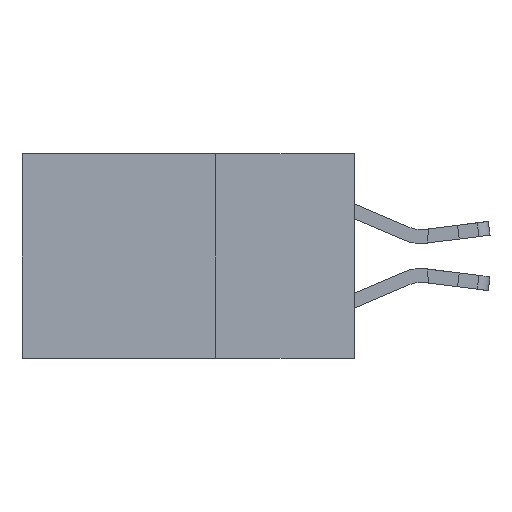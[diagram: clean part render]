
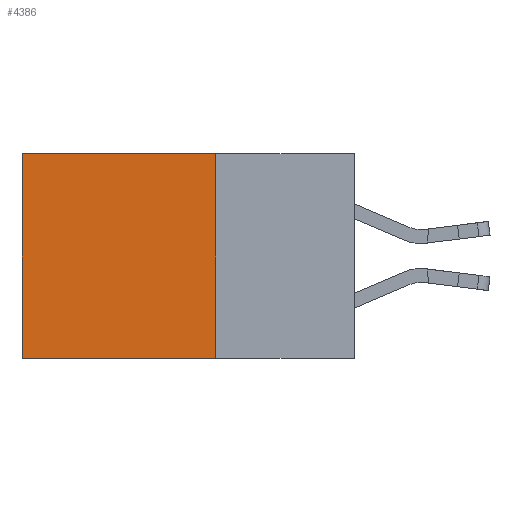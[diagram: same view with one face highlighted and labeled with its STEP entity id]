
A CAD part, left-side view. The second image highlights one B-rep face of the part: STEP entity #4386.
In plain terms, the highlighted planar face has unit normal (-1, 0, 0).
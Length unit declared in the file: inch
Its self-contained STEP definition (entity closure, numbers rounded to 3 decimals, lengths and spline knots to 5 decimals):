
#367 = DIRECTION ( 'NONE',  ( 0., 0., -1. ) ) ;
#418 = AXIS2_PLACEMENT_3D ( 'NONE', #9059, #8296, #367 ) ;
#1552 = DIRECTION ( 'NONE',  ( 0., 0., -1. ) ) ;
#1783 = LINE ( 'NONE', #6943, #2686 ) ;
#2231 = CARTESIAN_POINT ( 'NONE',  ( 0.2615, 0.25, -0.37 ) ) ;
#2245 = LINE ( 'NONE', #2784, #10789 ) ;
#2415 = CARTESIAN_POINT ( 'NONE',  ( 0.2615, 0.6, -0.37 ) ) ;
#2583 = VECTOR ( 'NONE', #1552, 39.37008 ) ;
#2585 = VERTEX_POINT ( 'NONE', #7213 ) ;
#2609 = EDGE_CURVE ( 'NONE', #7140, #4555, #1783, .T. ) ;
#2686 = VECTOR ( 'NONE', #7809, 39.37008 ) ;
#2784 = CARTESIAN_POINT ( 'NONE',  ( 0.2615, 0.25, -0.37 ) ) ;
#3113 = LINE ( 'NONE', #2231, #7549 ) ;
#3255 = CARTESIAN_POINT ( 'NONE',  ( 0.2615, 0.25, 0. ) ) ;
#3738 = ORIENTED_EDGE ( 'NONE', *, *, #10870, .F. ) ;
#4386 = ADVANCED_FACE ( 'NONE', ( #9820 ), #7427, .F. ) ;
#4390 = ORIENTED_EDGE ( 'NONE', *, *, #2609, .T. ) ;
#4555 = VERTEX_POINT ( 'NONE', #4958 ) ;
#4958 = CARTESIAN_POINT ( 'NONE',  ( 0.2615, 0.6, 0. ) ) ;
#5749 = VERTEX_POINT ( 'NONE', #9417 ) ;
#6943 = CARTESIAN_POINT ( 'NONE',  ( 0.2615, 0.25, 0. ) ) ;
#7140 = VERTEX_POINT ( 'NONE', #3255 ) ;
#7213 = CARTESIAN_POINT ( 'NONE',  ( 0.2615, 0.6, -0.37 ) ) ;
#7427 = PLANE ( 'NONE',  #418 ) ;
#7490 = ORIENTED_EDGE ( 'NONE', *, *, #10914, .T. ) ;
#7549 = VECTOR ( 'NONE', #9359, 39.37008 ) ;
#7809 = DIRECTION ( 'NONE',  ( 0., 1., 0. ) ) ;
#8188 = EDGE_CURVE ( 'NONE', #7140, #5749, #2245, .T. ) ;
#8296 = DIRECTION ( 'NONE',  ( 1., 0., 0. ) ) ;
#8417 = ORIENTED_EDGE ( 'NONE', *, *, #8188, .F. ) ;
#9059 = CARTESIAN_POINT ( 'NONE',  ( 0.2615, 0.25, -0.37 ) ) ;
#9359 = DIRECTION ( 'NONE',  ( 0., 1., 0. ) ) ;
#9415 = LINE ( 'NONE', #2415, #2583 ) ;
#9417 = CARTESIAN_POINT ( 'NONE',  ( 0.2615, 0.25, -0.37 ) ) ;
#9732 = DIRECTION ( 'NONE',  ( 0., 0., -1. ) ) ;
#9820 = FACE_OUTER_BOUND ( 'NONE', #10651, .T. ) ;
#10651 = EDGE_LOOP ( 'NONE', ( #7490, #3738, #8417, #4390 ) ) ;
#10789 = VECTOR ( 'NONE', #9732, 39.37008 ) ;
#10870 = EDGE_CURVE ( 'NONE', #5749, #2585, #3113, .T. ) ;
#10914 = EDGE_CURVE ( 'NONE', #4555, #2585, #9415, .T. ) ;
